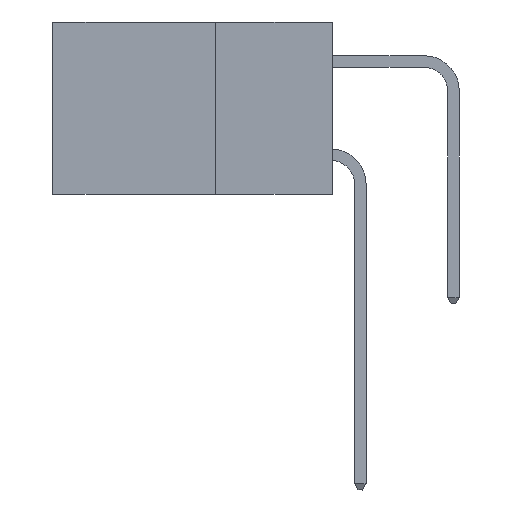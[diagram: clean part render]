
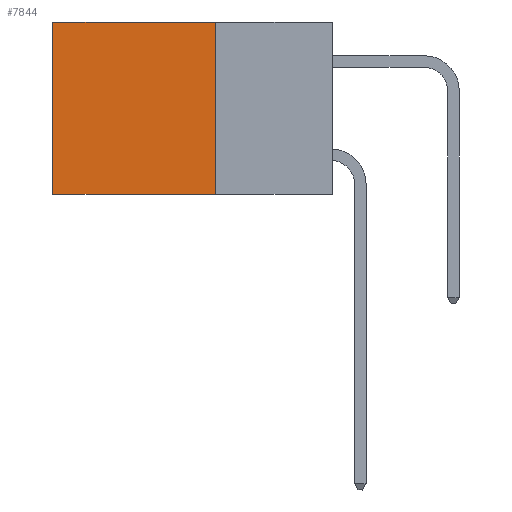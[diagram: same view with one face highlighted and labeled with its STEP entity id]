
A CAD part, left-side view. The second image highlights one B-rep face of the part: STEP entity #7844.
In plain terms, the highlighted planar face has unit normal (-1, 0, 0).
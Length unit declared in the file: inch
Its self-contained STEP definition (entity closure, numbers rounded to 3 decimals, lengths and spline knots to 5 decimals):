
#155 = VECTOR ( 'NONE', #2648, 39.37008 ) ;
#558 = VERTEX_POINT ( 'NONE', #6311 ) ;
#835 = DIRECTION ( 'NONE',  ( 1., 0., 0. ) ) ;
#1085 = EDGE_CURVE ( 'NONE', #9215, #2623, #10500, .T. ) ;
#1690 = VECTOR ( 'NONE', #6041, 39.37008 ) ;
#1783 = CARTESIAN_POINT ( 'NONE',  ( 0.2615, 0.25, 0. ) ) ;
#2337 = EDGE_LOOP ( 'NONE', ( #7402, #6894, #3752, #10035 ) ) ;
#2614 = DIRECTION ( 'NONE',  ( 0., 0., -1. ) ) ;
#2623 = VERTEX_POINT ( 'NONE', #11120 ) ;
#2648 = DIRECTION ( 'NONE',  ( 0., 1., 0. ) ) ;
#3646 = EDGE_CURVE ( 'NONE', #2623, #558, #4285, .T. ) ;
#3684 = CARTESIAN_POINT ( 'NONE',  ( 0.2615, 0.25, -0.37 ) ) ;
#3752 = ORIENTED_EDGE ( 'NONE', *, *, #5443, .F. ) ;
#3893 = VECTOR ( 'NONE', #6265, 39.37008 ) ;
#4285 = LINE ( 'NONE', #9553, #1690 ) ;
#4441 = PLANE ( 'NONE',  #9766 ) ;
#4586 = VECTOR ( 'NONE', #4717, 39.37008 ) ;
#4717 = DIRECTION ( 'NONE',  ( 0., 0., -1. ) ) ;
#5178 = VERTEX_POINT ( 'NONE', #7525 ) ;
#5443 = EDGE_CURVE ( 'NONE', #9215, #5178, #6544, .T. ) ;
#6041 = DIRECTION ( 'NONE',  ( 0., 0., -1. ) ) ;
#6265 = DIRECTION ( 'NONE',  ( 0., 1., 0. ) ) ;
#6311 = CARTESIAN_POINT ( 'NONE',  ( 0.2615, 0.6, -0.37 ) ) ;
#6455 = EDGE_CURVE ( 'NONE', #5178, #558, #9711, .T. ) ;
#6544 = LINE ( 'NONE', #10898, #4586 ) ;
#6894 = ORIENTED_EDGE ( 'NONE', *, *, #6455, .F. ) ;
#6966 = FACE_OUTER_BOUND ( 'NONE', #2337, .T. ) ;
#7402 = ORIENTED_EDGE ( 'NONE', *, *, #3646, .T. ) ;
#7525 = CARTESIAN_POINT ( 'NONE',  ( 0.2615, 0.25, -0.37 ) ) ;
#7844 = ADVANCED_FACE ( 'NONE', ( #6966 ), #4441, .F. ) ;
#9137 = CARTESIAN_POINT ( 'NONE',  ( 0.2615, 0.25, 0. ) ) ;
#9215 = VERTEX_POINT ( 'NONE', #9137 ) ;
#9553 = CARTESIAN_POINT ( 'NONE',  ( 0.2615, 0.6, -0.37 ) ) ;
#9711 = LINE ( 'NONE', #3684, #3893 ) ;
#9766 = AXIS2_PLACEMENT_3D ( 'NONE', #10471, #835, #2614 ) ;
#10035 = ORIENTED_EDGE ( 'NONE', *, *, #1085, .T. ) ;
#10471 = CARTESIAN_POINT ( 'NONE',  ( 0.2615, 0.25, -0.37 ) ) ;
#10500 = LINE ( 'NONE', #1783, #155 ) ;
#10898 = CARTESIAN_POINT ( 'NONE',  ( 0.2615, 0.25, -0.37 ) ) ;
#11120 = CARTESIAN_POINT ( 'NONE',  ( 0.2615, 0.6, 0. ) ) ;
